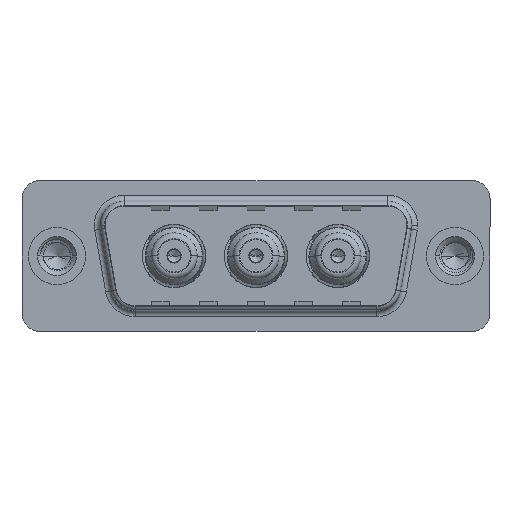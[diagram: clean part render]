
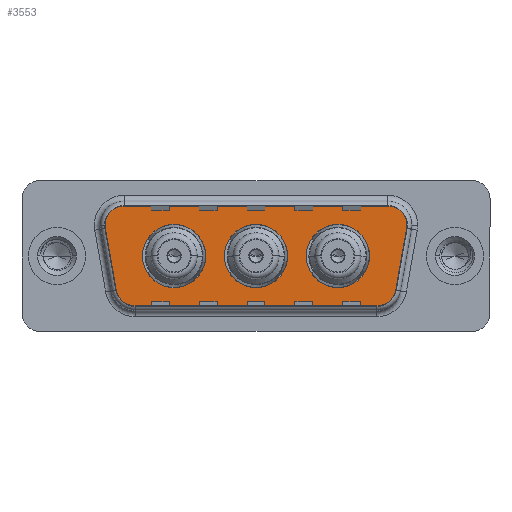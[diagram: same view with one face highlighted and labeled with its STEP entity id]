
A CAD part, top view. The second image highlights one B-rep face of the part: STEP entity #3553.
In plain terms, the highlighted planar face has unit normal (0, 0, 1).
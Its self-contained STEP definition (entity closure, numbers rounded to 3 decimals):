
#64 = DIRECTION ( 'NONE',  ( 1., 0., 0. ) ) ;
#80 = ORIENTED_EDGE ( 'NONE', *, *, #3100, .F. ) ;
#377 = CARTESIAN_POINT ( 'NONE',  ( 16.65, 0., 0. ) ) ;
#442 = CIRCLE ( 'NONE', #6236, 2.65 ) ;
#452 = VERTEX_POINT ( 'NONE', #14747 ) ;
#576 = CIRCLE ( 'NONE', #4924, 2.65 ) ;
#747 = CARTESIAN_POINT ( 'NONE',  ( 27.889, 4.9, 0. ) ) ;
#813 = EDGE_CURVE ( 'NONE', #16704, #18175, #4914, .T. ) ;
#820 = EDGE_LOOP ( 'NONE', ( #19897, #80 ) ) ;
#1118 = EDGE_CURVE ( 'NONE', #15438, #8281, #14568, .T. ) ;
#1121 = VECTOR ( 'NONE', #9531, 1000. ) ;
#1303 = CARTESIAN_POINT ( 'NONE',  ( 26.866, -2.9, 0. ) ) ;
#1365 = ORIENTED_EDGE ( 'NONE', *, *, #18154, .F. ) ;
#1419 = CARTESIAN_POINT ( 'NONE',  ( 5.411, 4.9, 0. ) ) ;
#1930 = CIRCLE ( 'NONE', #15345, 2. ) ;
#2324 = EDGE_CURVE ( 'NONE', #20155, #7894, #1930, .T. ) ;
#2375 = FACE_BOUND ( 'NONE', #13619, .T. ) ;
#2403 = EDGE_CURVE ( 'NONE', #8281, #11892, #17252, .T. ) ;
#2436 = CARTESIAN_POINT ( 'NONE',  ( 29.859, 2.553, 0. ) ) ;
#2773 = DIRECTION ( 'NONE',  ( 0., 0., 1. ) ) ;
#2779 = CIRCLE ( 'NONE', #15792, 2. ) ;
#2944 = CARTESIAN_POINT ( 'NONE',  ( 26.866, -2.9, 0. ) ) ;
#3085 = LINE ( 'NONE', #6130, #16199 ) ;
#3100 = EDGE_CURVE ( 'NONE', #14018, #12461, #3624, .T. ) ;
#3235 = CIRCLE ( 'NONE', #6403, 2. ) ;
#3358 = ORIENTED_EDGE ( 'NONE', *, *, #2403, .T. ) ;
#3553 = ADVANCED_FACE ( 'NONE', ( #18174, #2375, #5615, #10300 ), #18262, .T. ) ;
#3624 = CIRCLE ( 'NONE', #8896, 2.65 ) ;
#3806 = DIRECTION ( 'NONE',  ( -1., 0., 0. ) ) ;
#3867 = CARTESIAN_POINT ( 'NONE',  ( 14., 0., 0. ) ) ;
#4285 = DIRECTION ( 'NONE',  ( 0., 0., 1. ) ) ;
#4618 = EDGE_LOOP ( 'NONE', ( #8758, #8054 ) ) ;
#4748 = CARTESIAN_POINT ( 'NONE',  ( 7.15, 0., 0. ) ) ;
#4822 = CARTESIAN_POINT ( 'NONE',  ( 16.65, 0., 0. ) ) ;
#4914 = CIRCLE ( 'NONE', #10690, 2. ) ;
#4924 = AXIS2_PLACEMENT_3D ( 'NONE', #6136, #14233, #14955 ) ;
#4980 = CARTESIAN_POINT ( 'NONE',  ( 26.866, -4.9, 0. ) ) ;
#5166 = CARTESIAN_POINT ( 'NONE',  ( 3.441, 2.553, 0. ) ) ;
#5615 = FACE_BOUND ( 'NONE', #4618, .T. ) ;
#5912 = EDGE_CURVE ( 'NONE', #19840, #19368, #576, .T. ) ;
#5999 = EDGE_CURVE ( 'NONE', #13567, #452, #11209, .T. ) ;
#6130 = CARTESIAN_POINT ( 'NONE',  ( 29.859, 2.553, 0. ) ) ;
#6136 = CARTESIAN_POINT ( 'NONE',  ( 9.8, 0., 0. ) ) ;
#6161 = ORIENTED_EDGE ( 'NONE', *, *, #2324, .T. ) ;
#6236 = AXIS2_PLACEMENT_3D ( 'NONE', #18988, #9575, #64 ) ;
#6268 = DIRECTION ( 'NONE',  ( 1., 0., 0. ) ) ;
#6403 = AXIS2_PLACEMENT_3D ( 'NONE', #12265, #2773, #13836 ) ;
#6406 = DIRECTION ( 'NONE',  ( 1., 0., 0. ) ) ;
#6453 = ORIENTED_EDGE ( 'NONE', *, *, #15524, .T. ) ;
#6538 = DIRECTION ( 'NONE',  ( 0., 0., 1. ) ) ;
#6583 = EDGE_CURVE ( 'NONE', #11892, #13510, #2779, .T. ) ;
#6684 = DIRECTION ( 'NONE',  ( 1., 0., 0. ) ) ;
#6787 = DIRECTION ( 'NONE',  ( 0., 0., 1. ) ) ;
#7037 = CARTESIAN_POINT ( 'NONE',  ( 5.411, 2.9, 0. ) ) ;
#7099 = AXIS2_PLACEMENT_3D ( 'NONE', #4822, #15884, #6406 ) ;
#7445 = CARTESIAN_POINT ( 'NONE',  ( 26.15, 0., 0. ) ) ;
#7729 = DIRECTION ( 'NONE',  ( 0.174, 0.985, 0. ) ) ;
#7738 = CARTESIAN_POINT ( 'NONE',  ( 27.889, 2.9, 0. ) ) ;
#7845 = EDGE_CURVE ( 'NONE', #7894, #12800, #3235, .T. ) ;
#7894 = VERTEX_POINT ( 'NONE', #17068 ) ;
#7950 = CARTESIAN_POINT ( 'NONE',  ( 6.434, -4.9, 0. ) ) ;
#8054 = ORIENTED_EDGE ( 'NONE', *, *, #5912, .F. ) ;
#8121 = EDGE_CURVE ( 'NONE', #12461, #14018, #19282, .T. ) ;
#8281 = VERTEX_POINT ( 'NONE', #5166 ) ;
#8348 = CARTESIAN_POINT ( 'NONE',  ( 5.411, 4.9, 0. ) ) ;
#8358 = DIRECTION ( 'NONE',  ( 0., 0., 1. ) ) ;
#8405 = CARTESIAN_POINT ( 'NONE',  ( 3.441, 2.553, 0. ) ) ;
#8421 = CARTESIAN_POINT ( 'NONE',  ( 23.5, 0., 0. ) ) ;
#8634 = LINE ( 'NONE', #1419, #9131 ) ;
#8758 = ORIENTED_EDGE ( 'NONE', *, *, #15264, .F. ) ;
#8769 = CARTESIAN_POINT ( 'NONE',  ( 23.5, 0., 0. ) ) ;
#8784 = CARTESIAN_POINT ( 'NONE',  ( 6.434, -4.9, 0. ) ) ;
#8888 = VECTOR ( 'NONE', #12845, 1000. ) ;
#8896 = AXIS2_PLACEMENT_3D ( 'NONE', #377, #17966, #12494 ) ;
#9131 = VECTOR ( 'NONE', #12500, 1000. ) ;
#9246 = ORIENTED_EDGE ( 'NONE', *, *, #5999, .F. ) ;
#9258 = AXIS2_PLACEMENT_3D ( 'NONE', #7037, #6787, #6684 ) ;
#9292 = ORIENTED_EDGE ( 'NONE', *, *, #17746, .T. ) ;
#9531 = DIRECTION ( 'NONE',  ( 1., 0., 0. ) ) ;
#9575 = DIRECTION ( 'NONE',  ( 0., 0., 1. ) ) ;
#9782 = ORIENTED_EDGE ( 'NONE', *, *, #19185, .T. ) ;
#9796 = DIRECTION ( 'NONE',  ( 1., 0., 0. ) ) ;
#9885 = ORIENTED_EDGE ( 'NONE', *, *, #6583, .T. ) ;
#10108 = EDGE_LOOP ( 'NONE', ( #10736, #9292, #6161, #10817, #6453, #17752, #3358, #9885, #9782 ) ) ;
#10300 = FACE_OUTER_BOUND ( 'NONE', #10108, .T. ) ;
#10325 = DIRECTION ( 'NONE',  ( 1., 0., 0. ) ) ;
#10690 = AXIS2_PLACEMENT_3D ( 'NONE', #2944, #6538, #20312 ) ;
#10736 = ORIENTED_EDGE ( 'NONE', *, *, #813, .T. ) ;
#10781 = AXIS2_PLACEMENT_3D ( 'NONE', #8769, #19757, #10325 ) ;
#10817 = ORIENTED_EDGE ( 'NONE', *, *, #7845, .T. ) ;
#11209 = CIRCLE ( 'NONE', #14477, 2.65 ) ;
#11246 = AXIS2_PLACEMENT_3D ( 'NONE', #1303, #17787, #9796 ) ;
#11390 = CARTESIAN_POINT ( 'NONE',  ( 12.45, 0., 0. ) ) ;
#11892 = VERTEX_POINT ( 'NONE', #19128 ) ;
#12265 = CARTESIAN_POINT ( 'NONE',  ( 27.889, 2.9, 0. ) ) ;
#12461 = VERTEX_POINT ( 'NONE', #20299 ) ;
#12494 = DIRECTION ( 'NONE',  ( 1., 0., 0. ) ) ;
#12500 = DIRECTION ( 'NONE',  ( -1., 0., 0. ) ) ;
#12800 = VERTEX_POINT ( 'NONE', #747 ) ;
#12845 = DIRECTION ( 'NONE',  ( 0.174, -0.985, 0. ) ) ;
#13247 = DIRECTION ( 'NONE',  ( -1., 0., 0. ) ) ;
#13510 = VERTEX_POINT ( 'NONE', #8784 ) ;
#13567 = VERTEX_POINT ( 'NONE', #7445 ) ;
#13619 = EDGE_LOOP ( 'NONE', ( #9246, #1365 ) ) ;
#13743 = LINE ( 'NONE', #7950, #1121 ) ;
#13805 = DIRECTION ( 'NONE',  ( 0., 0., 1. ) ) ;
#13810 = CARTESIAN_POINT ( 'NONE',  ( 6.434, -2.9, 0. ) ) ;
#13836 = DIRECTION ( 'NONE',  ( -1., 0., 0. ) ) ;
#13971 = CIRCLE ( 'NONE', #10781, 2.65 ) ;
#14018 = VERTEX_POINT ( 'NONE', #3867 ) ;
#14233 = DIRECTION ( 'NONE',  ( 0., 0., 1. ) ) ;
#14477 = AXIS2_PLACEMENT_3D ( 'NONE', #8421, #8358, #6268 ) ;
#14568 = CIRCLE ( 'NONE', #9258, 2. ) ;
#14747 = CARTESIAN_POINT ( 'NONE',  ( 20.85, 0., 0. ) ) ;
#14955 = DIRECTION ( 'NONE',  ( 1., 0., 0. ) ) ;
#15108 = CARTESIAN_POINT ( 'NONE',  ( 28.836, -3.247, 0. ) ) ;
#15264 = EDGE_CURVE ( 'NONE', #19368, #19840, #442, .T. ) ;
#15345 = AXIS2_PLACEMENT_3D ( 'NONE', #7738, #4285, #3806 ) ;
#15438 = VERTEX_POINT ( 'NONE', #8348 ) ;
#15524 = EDGE_CURVE ( 'NONE', #12800, #15438, #8634, .T. ) ;
#15792 = AXIS2_PLACEMENT_3D ( 'NONE', #13810, #13805, #13247 ) ;
#15884 = DIRECTION ( 'NONE',  ( 0., 0., 1. ) ) ;
#16199 = VECTOR ( 'NONE', #7729, 1000. ) ;
#16704 = VERTEX_POINT ( 'NONE', #4980 ) ;
#17068 = CARTESIAN_POINT ( 'NONE',  ( 29.889, 2.9, 0. ) ) ;
#17252 = LINE ( 'NONE', #8405, #8888 ) ;
#17746 = EDGE_CURVE ( 'NONE', #18175, #20155, #3085, .T. ) ;
#17752 = ORIENTED_EDGE ( 'NONE', *, *, #1118, .T. ) ;
#17787 = DIRECTION ( 'NONE',  ( 0., 0., 1. ) ) ;
#17966 = DIRECTION ( 'NONE',  ( 0., 0., 1. ) ) ;
#18154 = EDGE_CURVE ( 'NONE', #452, #13567, #13971, .T. ) ;
#18174 = FACE_BOUND ( 'NONE', #820, .T. ) ;
#18175 = VERTEX_POINT ( 'NONE', #15108 ) ;
#18262 = PLANE ( 'NONE',  #11246 ) ;
#18988 = CARTESIAN_POINT ( 'NONE',  ( 9.8, 0., 0. ) ) ;
#19128 = CARTESIAN_POINT ( 'NONE',  ( 4.464, -3.247, 0. ) ) ;
#19185 = EDGE_CURVE ( 'NONE', #13510, #16704, #13743, .T. ) ;
#19282 = CIRCLE ( 'NONE', #7099, 2.65 ) ;
#19368 = VERTEX_POINT ( 'NONE', #11390 ) ;
#19757 = DIRECTION ( 'NONE',  ( 0., 0., 1. ) ) ;
#19840 = VERTEX_POINT ( 'NONE', #4748 ) ;
#19897 = ORIENTED_EDGE ( 'NONE', *, *, #8121, .F. ) ;
#20155 = VERTEX_POINT ( 'NONE', #2436 ) ;
#20299 = CARTESIAN_POINT ( 'NONE',  ( 19.3, 0., 0. ) ) ;
#20312 = DIRECTION ( 'NONE',  ( 1., 0., 0. ) ) ;
